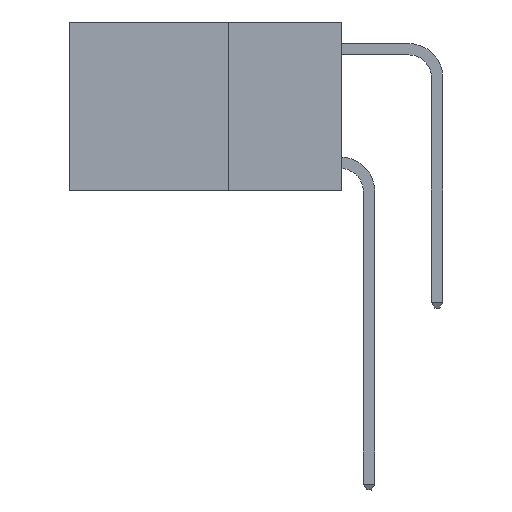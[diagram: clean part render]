
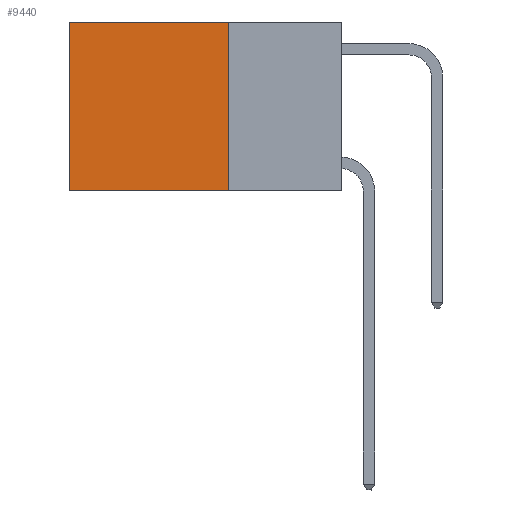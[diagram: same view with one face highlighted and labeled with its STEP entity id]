
A CAD part, left-side view. The second image highlights one B-rep face of the part: STEP entity #9440.
In plain terms, the highlighted planar face has unit normal (-1, 0, 0).
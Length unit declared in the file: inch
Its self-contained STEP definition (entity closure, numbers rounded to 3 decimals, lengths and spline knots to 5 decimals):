
#125 = DIRECTION ( 'NONE',  ( 0., 0., -1. ) ) ;
#519 = CARTESIAN_POINT ( 'NONE',  ( 0.2625, 0.25, 0. ) ) ;
#1047 = PLANE ( 'NONE',  #6719 ) ;
#1261 = CARTESIAN_POINT ( 'NONE',  ( 0.2625, 0.25, -0.37 ) ) ;
#1290 = LINE ( 'NONE', #1261, #12966 ) ;
#2251 = VERTEX_POINT ( 'NONE', #4200 ) ;
#2329 = VECTOR ( 'NONE', #12935, 39.37008 ) ;
#3134 = ORIENTED_EDGE ( 'NONE', *, *, #3203, .T. ) ;
#3136 = ORIENTED_EDGE ( 'NONE', *, *, #4801, .F. ) ;
#3203 = EDGE_CURVE ( 'NONE', #12999, #2251, #4802, .T. ) ;
#3362 = DIRECTION ( 'NONE',  ( 1., 0., 0. ) ) ;
#3531 = DIRECTION ( 'NONE',  ( 0., 1., 0. ) ) ;
#3895 = CARTESIAN_POINT ( 'NONE',  ( 0.2625, 0.25, 0. ) ) ;
#3910 = VERTEX_POINT ( 'NONE', #4703 ) ;
#4077 = EDGE_LOOP ( 'NONE', ( #3134, #14047, #3136, #13182 ) ) ;
#4200 = CARTESIAN_POINT ( 'NONE',  ( 0.2625, 0.6, -0.37 ) ) ;
#4574 = EDGE_CURVE ( 'NONE', #14517, #12999, #11590, .T. ) ;
#4703 = CARTESIAN_POINT ( 'NONE',  ( 0.2625, 0.25, -0.37 ) ) ;
#4720 = CARTESIAN_POINT ( 'NONE',  ( 0.2625, 0.6, 0. ) ) ;
#4801 = EDGE_CURVE ( 'NONE', #14517, #3910, #5677, .T. ) ;
#4802 = LINE ( 'NONE', #4720, #13468 ) ;
#5677 = LINE ( 'NONE', #3895, #2329 ) ;
#5787 = FACE_OUTER_BOUND ( 'NONE', #4077, .T. ) ;
#6719 = AXIS2_PLACEMENT_3D ( 'NONE', #10183, #3362, #11305 ) ;
#7028 = EDGE_CURVE ( 'NONE', #3910, #2251, #1290, .T. ) ;
#8144 = CARTESIAN_POINT ( 'NONE',  ( 0.2625, 0.6, 0. ) ) ;
#8329 = VECTOR ( 'NONE', #3531, 39.37008 ) ;
#9264 = CARTESIAN_POINT ( 'NONE',  ( 0.2625, 0.25, 0. ) ) ;
#9440 = ADVANCED_FACE ( 'NONE', ( #5787 ), #1047, .F. ) ;
#10183 = CARTESIAN_POINT ( 'NONE',  ( 0.2625, 0.25, 0. ) ) ;
#11305 = DIRECTION ( 'NONE',  ( 0., 0., -1. ) ) ;
#11509 = DIRECTION ( 'NONE',  ( 0., 1., 0. ) ) ;
#11590 = LINE ( 'NONE', #9264, #8329 ) ;
#12935 = DIRECTION ( 'NONE',  ( 0., 0., -1. ) ) ;
#12966 = VECTOR ( 'NONE', #11509, 39.37008 ) ;
#12999 = VERTEX_POINT ( 'NONE', #8144 ) ;
#13182 = ORIENTED_EDGE ( 'NONE', *, *, #4574, .T. ) ;
#13468 = VECTOR ( 'NONE', #125, 39.37008 ) ;
#14047 = ORIENTED_EDGE ( 'NONE', *, *, #7028, .F. ) ;
#14517 = VERTEX_POINT ( 'NONE', #519 ) ;
